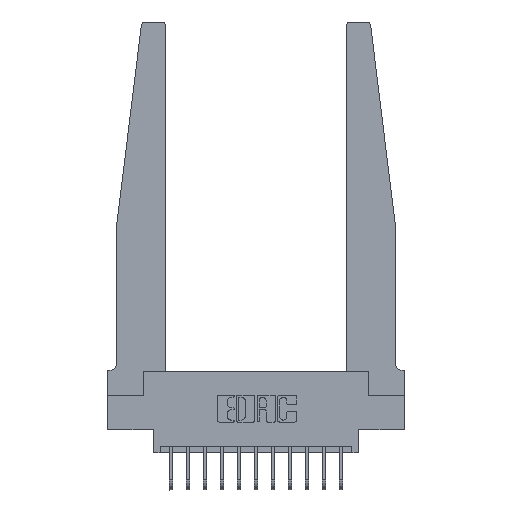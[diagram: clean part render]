
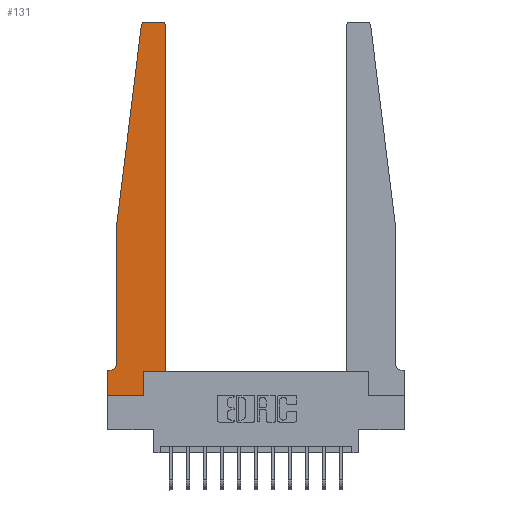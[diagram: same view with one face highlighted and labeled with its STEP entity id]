
A CAD part, top view. The second image highlights one B-rep face of the part: STEP entity #131.
In plain terms, the highlighted planar face has unit normal (0, 0, 1).
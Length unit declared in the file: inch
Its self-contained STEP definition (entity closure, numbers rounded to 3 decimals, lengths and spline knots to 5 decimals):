
#131 = ADVANCED_FACE ( 'NONE', ( #1412 ), #5756, .T. ) ;
#282 = DIRECTION ( 'NONE',  ( -1., 0., 0. ) ) ;
#522 = VERTEX_POINT ( 'NONE', #17117 ) ;
#563 = ORIENTED_EDGE ( 'NONE', *, *, #12236, .T. ) ;
#657 = CARTESIAN_POINT ( 'NONE',  ( 0.395, 2.72, 0.37 ) ) ;
#721 = ORIENTED_EDGE ( 'NONE', *, *, #16698, .T. ) ;
#787 = ORIENTED_EDGE ( 'NONE', *, *, #2724, .T. ) ;
#926 = LINE ( 'NONE', #14960, #3587 ) ;
#1014 = DIRECTION ( 'NONE',  ( 0., -1., 0. ) ) ;
#1029 = CIRCLE ( 'NONE', #16549, 0.03 ) ;
#1086 = EDGE_CURVE ( 'NONE', #17451, #16619, #16814, .T. ) ;
#1149 = VECTOR ( 'NONE', #11069, 39.37008 ) ;
#1151 = CARTESIAN_POINT ( 'NONE',  ( 0., 0.1875, 0.37 ) ) ;
#1412 = FACE_OUTER_BOUND ( 'NONE', #1811, .T. ) ;
#1527 = CIRCLE ( 'NONE', #14993, 0.05 ) ;
#1630 = EDGE_CURVE ( 'NONE', #2458, #1941, #13484, .T. ) ;
#1811 = EDGE_LOOP ( 'NONE', ( #10749, #787, #721, #6323, #7051, #7394, #12993, #13078, #7047, #10972, #10723, #563 ) ) ;
#1846 = DIRECTION ( 'NONE',  ( 1., 0., 0. ) ) ;
#1941 = VERTEX_POINT ( 'NONE', #6335 ) ;
#2118 = DIRECTION ( 'NONE',  ( 1., 0., 0. ) ) ;
#2263 = CARTESIAN_POINT ( 'NONE',  ( 0.2605, 0.18, 0.37 ) ) ;
#2458 = VERTEX_POINT ( 'NONE', #6594 ) ;
#2605 = EDGE_CURVE ( 'NONE', #522, #5039, #7114, .T. ) ;
#2724 = EDGE_CURVE ( 'NONE', #16656, #15565, #8588, .T. ) ;
#2959 = CARTESIAN_POINT ( 'NONE',  ( 0.015, 0.2375, 0.37 ) ) ;
#3577 = EDGE_CURVE ( 'NONE', #16619, #17517, #926, .T. ) ;
#3587 = VECTOR ( 'NONE', #2118, 39.37008 ) ;
#4424 = VECTOR ( 'NONE', #1014, 39.37008 ) ;
#4571 = CARTESIAN_POINT ( 'NONE',  ( 0.065, 0.2375, 0.37 ) ) ;
#5039 = VERTEX_POINT ( 'NONE', #4571 ) ;
#5148 = CARTESIAN_POINT ( 'NONE',  ( 0., 0., 0.37 ) ) ;
#5333 = CARTESIAN_POINT ( 'NONE',  ( 0.065, 1.25, 0.37 ) ) ;
#5478 = EDGE_CURVE ( 'NONE', #16931, #16656, #14607, .T. ) ;
#5482 = CARTESIAN_POINT ( 'NONE',  ( 0.425, 2.72, 0.37 ) ) ;
#5631 = CARTESIAN_POINT ( 'NONE',  ( 0.015, 0.1875, 0.37 ) ) ;
#5756 = PLANE ( 'NONE',  #15144 ) ;
#5850 = VECTOR ( 'NONE', #13456, 39.37008 ) ;
#6123 = DIRECTION ( 'NONE',  ( 0., 0., -1. ) ) ;
#6323 = ORIENTED_EDGE ( 'NONE', *, *, #2605, .T. ) ;
#6335 = CARTESIAN_POINT ( 'NONE',  ( 0.425, 0.18, 0.37 ) ) ;
#6594 = CARTESIAN_POINT ( 'NONE',  ( 0.2605, 0.18, 0.37 ) ) ;
#7047 = ORIENTED_EDGE ( 'NONE', *, *, #12868, .T. ) ;
#7051 = ORIENTED_EDGE ( 'NONE', *, *, #7759, .T. ) ;
#7114 = LINE ( 'NONE', #9683, #13635 ) ;
#7218 = CARTESIAN_POINT ( 'NONE',  ( 0.425, 0.18, 0.37 ) ) ;
#7394 = ORIENTED_EDGE ( 'NONE', *, *, #12738, .T. ) ;
#7598 = CARTESIAN_POINT ( 'NONE',  ( 0.2605, 0., 0.37 ) ) ;
#7759 = EDGE_CURVE ( 'NONE', #5039, #17851, #1527, .T. ) ;
#8048 = DIRECTION ( 'NONE',  ( 0., 1., 0. ) ) ;
#8265 = DIRECTION ( 'NONE',  ( 0., -1., 0. ) ) ;
#8588 = CIRCLE ( 'NONE', #13038, 0.03 ) ;
#9022 = CARTESIAN_POINT ( 'NONE',  ( 0.425, 0.18, 0.37 ) ) ;
#9683 = CARTESIAN_POINT ( 'NONE',  ( 0.065, 1.25, 0.37 ) ) ;
#10364 = DIRECTION ( 'NONE',  ( 0., 0., 1. ) ) ;
#10629 = VECTOR ( 'NONE', #8048, 39.37008 ) ;
#10723 = ORIENTED_EDGE ( 'NONE', *, *, #14883, .T. ) ;
#10749 = ORIENTED_EDGE ( 'NONE', *, *, #5478, .T. ) ;
#10866 = LINE ( 'NONE', #2263, #10629 ) ;
#10972 = ORIENTED_EDGE ( 'NONE', *, *, #1630, .T. ) ;
#11069 = DIRECTION ( 'NONE',  ( -0.122, -0.992, 0. ) ) ;
#11220 = VERTEX_POINT ( 'NONE', #5482 ) ;
#11478 = DIRECTION ( 'NONE',  ( 0., 0., 1. ) ) ;
#11794 = CARTESIAN_POINT ( 'NONE',  ( 0.065, 0.1875, 0.37 ) ) ;
#11809 = CARTESIAN_POINT ( 'NONE',  ( 0.25, 2.75, 0.37 ) ) ;
#12236 = EDGE_CURVE ( 'NONE', #11220, #16931, #1029, .T. ) ;
#12266 = CARTESIAN_POINT ( 'NONE',  ( 0.27653, 2.75, 0.37 ) ) ;
#12455 = DIRECTION ( 'NONE',  ( 1., 0., 0. ) ) ;
#12738 = EDGE_CURVE ( 'NONE', #17851, #17451, #14856, .T. ) ;
#12868 = EDGE_CURVE ( 'NONE', #17517, #2458, #10866, .T. ) ;
#12920 = DIRECTION ( 'NONE',  ( 0., 1., 0. ) ) ;
#12993 = ORIENTED_EDGE ( 'NONE', *, *, #1086, .T. ) ;
#13038 = AXIS2_PLACEMENT_3D ( 'NONE', #18212, #10364, #16112 ) ;
#13078 = ORIENTED_EDGE ( 'NONE', *, *, #3577, .T. ) ;
#13100 = DIRECTION ( 'NONE',  ( -1., 0., 0. ) ) ;
#13456 = DIRECTION ( 'NONE',  ( -1., 0., 0. ) ) ;
#13475 = DIRECTION ( 'NONE',  ( 0., 0., 1. ) ) ;
#13484 = LINE ( 'NONE', #9022, #16343 ) ;
#13635 = VECTOR ( 'NONE', #8265, 39.37008 ) ;
#14348 = LINE ( 'NONE', #7218, #15791 ) ;
#14607 = LINE ( 'NONE', #11809, #16638 ) ;
#14856 = LINE ( 'NONE', #11794, #5850 ) ;
#14883 = EDGE_CURVE ( 'NONE', #1941, #11220, #14348, .T. ) ;
#14960 = CARTESIAN_POINT ( 'NONE',  ( 0., 0., 0.37 ) ) ;
#14993 = AXIS2_PLACEMENT_3D ( 'NONE', #2959, #6123, #13100 ) ;
#15144 = AXIS2_PLACEMENT_3D ( 'NONE', #1151, #11478, #17136 ) ;
#15397 = CARTESIAN_POINT ( 'NONE',  ( 0.395, 2.75, 0.37 ) ) ;
#15565 = VERTEX_POINT ( 'NONE', #17168 ) ;
#15791 = VECTOR ( 'NONE', #12920, 39.37008 ) ;
#16112 = DIRECTION ( 'NONE',  ( 1., 0., 0. ) ) ;
#16343 = VECTOR ( 'NONE', #1846, 39.37008 ) ;
#16549 = AXIS2_PLACEMENT_3D ( 'NONE', #657, #13475, #12455 ) ;
#16610 = CARTESIAN_POINT ( 'NONE',  ( 0., 0., 0.37 ) ) ;
#16619 = VERTEX_POINT ( 'NONE', #5148 ) ;
#16638 = VECTOR ( 'NONE', #282, 39.37008 ) ;
#16656 = VERTEX_POINT ( 'NONE', #12266 ) ;
#16698 = EDGE_CURVE ( 'NONE', #15565, #522, #18142, .T. ) ;
#16814 = LINE ( 'NONE', #16610, #4424 ) ;
#16931 = VERTEX_POINT ( 'NONE', #15397 ) ;
#17117 = CARTESIAN_POINT ( 'NONE',  ( 0.065, 1.25, 0.37 ) ) ;
#17136 = DIRECTION ( 'NONE',  ( 1., 0., 0. ) ) ;
#17168 = CARTESIAN_POINT ( 'NONE',  ( 0.24675, 2.72367, 0.37 ) ) ;
#17451 = VERTEX_POINT ( 'NONE', #17488 ) ;
#17488 = CARTESIAN_POINT ( 'NONE',  ( 0., 0.1875, 0.37 ) ) ;
#17517 = VERTEX_POINT ( 'NONE', #7598 ) ;
#17851 = VERTEX_POINT ( 'NONE', #5631 ) ;
#18142 = LINE ( 'NONE', #5333, #1149 ) ;
#18212 = CARTESIAN_POINT ( 'NONE',  ( 0.27653, 2.72, 0.37 ) ) ;
